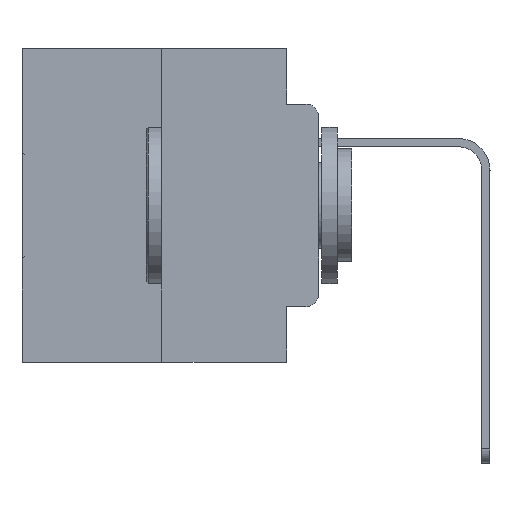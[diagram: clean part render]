
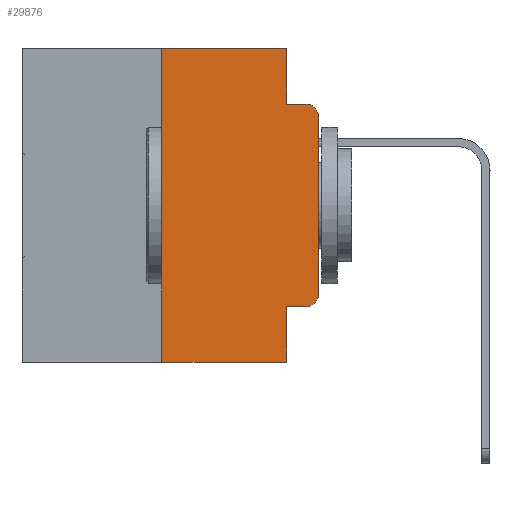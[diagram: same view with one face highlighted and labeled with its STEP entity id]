
A CAD part, left-side view. The second image highlights one B-rep face of the part: STEP entity #29876.
In plain terms, the highlighted planar face has unit normal (-1, 0, 0).
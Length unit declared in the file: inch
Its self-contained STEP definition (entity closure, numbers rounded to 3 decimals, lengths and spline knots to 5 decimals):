
#461 = DIRECTION ( 'NONE',  ( 0., 0., -1. ) ) ;
#485 = CARTESIAN_POINT ( 'NONE',  ( 0., 0.051, -0.4115 ) ) ;
#739 = PLANE ( 'NONE',  #24932 ) ;
#891 = EDGE_CURVE ( 'NONE', #8878, #20569, #20020, .T. ) ;
#1150 = DIRECTION ( 'NONE',  ( 0., -1., 0. ) ) ;
#1333 = EDGE_CURVE ( 'NONE', #3500, #28423, #12259, .T. ) ;
#1470 = LINE ( 'NONE', #17090, #7018 ) ;
#1945 = VERTEX_POINT ( 'NONE', #6977 ) ;
#2056 = EDGE_CURVE ( 'NONE', #8474, #2846, #1470, .T. ) ;
#2163 = LINE ( 'NONE', #20204, #26573 ) ;
#2752 = CARTESIAN_POINT ( 'NONE',  ( 0., 0.051, -0.0885 ) ) ;
#2813 = ORIENTED_EDGE ( 'NONE', *, *, #891, .F. ) ;
#2846 = VERTEX_POINT ( 'NONE', #17999 ) ;
#2902 = VECTOR ( 'NONE', #24839, 39.37008 ) ;
#3194 = ORIENTED_EDGE ( 'NONE', *, *, #2056, .T. ) ;
#3418 = EDGE_CURVE ( 'NONE', #9445, #8878, #10677, .T. ) ;
#3500 = VERTEX_POINT ( 'NONE', #30174 ) ;
#3915 = DIRECTION ( 'NONE',  ( 1., 0., 0. ) ) ;
#5936 = CARTESIAN_POINT ( 'NONE',  ( 0., 0.051, 0. ) ) ;
#6326 = DIRECTION ( 'NONE',  ( 0., 0., -1. ) ) ;
#6813 = CARTESIAN_POINT ( 'NONE',  ( 0., 0.02, -0.1085 ) ) ;
#6977 = CARTESIAN_POINT ( 'NONE',  ( 0., 0.02, -0.4115 ) ) ;
#7018 = VECTOR ( 'NONE', #14528, 39.37008 ) ;
#7470 = VECTOR ( 'NONE', #6326, 39.37008 ) ;
#8068 = LINE ( 'NONE', #26370, #8800 ) ;
#8474 = VERTEX_POINT ( 'NONE', #15907 ) ;
#8577 = DIRECTION ( 'NONE',  ( 0., 0., -1. ) ) ;
#8800 = VECTOR ( 'NONE', #461, 39.37008 ) ;
#8878 = VERTEX_POINT ( 'NONE', #5936 ) ;
#8911 = VECTOR ( 'NONE', #1150, 39.37008 ) ;
#8959 = ORIENTED_EDGE ( 'NONE', *, *, #1333, .T. ) ;
#9141 = CIRCLE ( 'NONE', #15188, 0.02 ) ;
#9389 = EDGE_CURVE ( 'NONE', #18680, #2846, #8068, .T. ) ;
#9445 = VERTEX_POINT ( 'NONE', #24404 ) ;
#10221 = ORIENTED_EDGE ( 'NONE', *, *, #9389, .F. ) ;
#10677 = LINE ( 'NONE', #15357, #2902 ) ;
#10786 = AXIS2_PLACEMENT_3D ( 'NONE', #22518, #13127, #8577 ) ;
#11579 = EDGE_LOOP ( 'NONE', ( #8959, #17249, #24102, #2813, #26624, #23514, #3194, #10221, #25373, #29237 ) ) ;
#12259 = LINE ( 'NONE', #24698, #30320 ) ;
#12718 = DIRECTION ( 'NONE',  ( 0., 0., 1. ) ) ;
#13127 = DIRECTION ( 'NONE',  ( -1., 0., 0. ) ) ;
#13241 = DIRECTION ( 'NONE',  ( 0., 0., 1. ) ) ;
#13260 = CARTESIAN_POINT ( 'NONE',  ( 0., 0.051, 0. ) ) ;
#13672 = EDGE_CURVE ( 'NONE', #1945, #3500, #14858, .T. ) ;
#13702 = EDGE_CURVE ( 'NONE', #18680, #1945, #15217, .T. ) ;
#14435 = CARTESIAN_POINT ( 'NONE',  ( 0., 0.051, -0.0885 ) ) ;
#14528 = DIRECTION ( 'NONE',  ( 0., -1., 0. ) ) ;
#14629 = EDGE_CURVE ( 'NONE', #8474, #9445, #2163, .T. ) ;
#14858 = CIRCLE ( 'NONE', #10786, 0.02 ) ;
#14991 = EDGE_CURVE ( 'NONE', #20569, #20060, #29849, .T. ) ;
#15188 = AXIS2_PLACEMENT_3D ( 'NONE', #6813, #30441, #20752 ) ;
#15217 = LINE ( 'NONE', #27162, #8911 ) ;
#15357 = CARTESIAN_POINT ( 'NONE',  ( 0., 0.473, 0. ) ) ;
#15907 = CARTESIAN_POINT ( 'NONE',  ( 0., 0.25, -0.5 ) ) ;
#16102 = EDGE_CURVE ( 'NONE', #28423, #20060, #9141, .T. ) ;
#17090 = CARTESIAN_POINT ( 'NONE',  ( 0., 0.473, -0.5 ) ) ;
#17249 = ORIENTED_EDGE ( 'NONE', *, *, #16102, .T. ) ;
#17751 = CARTESIAN_POINT ( 'NONE',  ( 0., 0.473, 0. ) ) ;
#17999 = CARTESIAN_POINT ( 'NONE',  ( 0., 0.051, -0.5 ) ) ;
#18680 = VERTEX_POINT ( 'NONE', #485 ) ;
#20020 = LINE ( 'NONE', #13260, #7470 ) ;
#20060 = VERTEX_POINT ( 'NONE', #26439 ) ;
#20204 = CARTESIAN_POINT ( 'NONE',  ( 0., 0.25, 0. ) ) ;
#20569 = VERTEX_POINT ( 'NONE', #2752 ) ;
#20752 = DIRECTION ( 'NONE',  ( 0., 0., -1. ) ) ;
#20996 = VECTOR ( 'NONE', #26187, 39.37008 ) ;
#22518 = CARTESIAN_POINT ( 'NONE',  ( 0., 0.02, -0.3915 ) ) ;
#23514 = ORIENTED_EDGE ( 'NONE', *, *, #14629, .F. ) ;
#24102 = ORIENTED_EDGE ( 'NONE', *, *, #14991, .F. ) ;
#24404 = CARTESIAN_POINT ( 'NONE',  ( 0., 0.25, 0. ) ) ;
#24698 = CARTESIAN_POINT ( 'NONE',  ( 0., 0., 0. ) ) ;
#24839 = DIRECTION ( 'NONE',  ( 0., -1., 0. ) ) ;
#24932 = AXIS2_PLACEMENT_3D ( 'NONE', #17751, #3915, #29923 ) ;
#25373 = ORIENTED_EDGE ( 'NONE', *, *, #13702, .T. ) ;
#26187 = DIRECTION ( 'NONE',  ( 0., -1., 0. ) ) ;
#26370 = CARTESIAN_POINT ( 'NONE',  ( 0., 0.051, 0. ) ) ;
#26439 = CARTESIAN_POINT ( 'NONE',  ( 0., 0.02, -0.0885 ) ) ;
#26573 = VECTOR ( 'NONE', #12718, 39.37008 ) ;
#26624 = ORIENTED_EDGE ( 'NONE', *, *, #3418, .F. ) ;
#27078 = FACE_OUTER_BOUND ( 'NONE', #11579, .T. ) ;
#27162 = CARTESIAN_POINT ( 'NONE',  ( 0., 0.051, -0.4115 ) ) ;
#27886 = CARTESIAN_POINT ( 'NONE',  ( 0., 0., -0.1085 ) ) ;
#28423 = VERTEX_POINT ( 'NONE', #27886 ) ;
#29237 = ORIENTED_EDGE ( 'NONE', *, *, #13672, .T. ) ;
#29849 = LINE ( 'NONE', #14435, #20996 ) ;
#29876 = ADVANCED_FACE ( 'NONE', ( #27078 ), #739, .F. ) ;
#29923 = DIRECTION ( 'NONE',  ( 0., 0., -1. ) ) ;
#30174 = CARTESIAN_POINT ( 'NONE',  ( 0., 0., -0.3915 ) ) ;
#30320 = VECTOR ( 'NONE', #13241, 39.37008 ) ;
#30441 = DIRECTION ( 'NONE',  ( -1., 0., 0. ) ) ;
